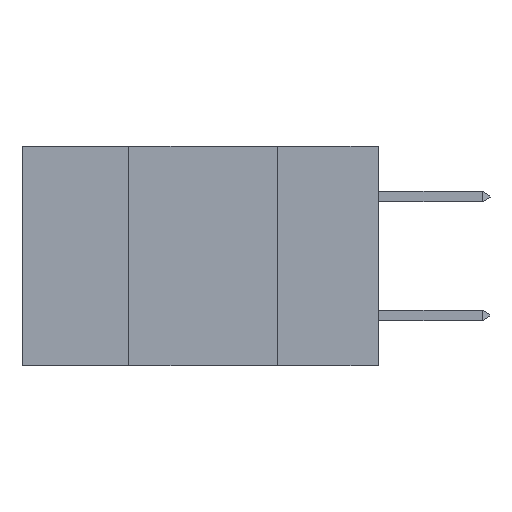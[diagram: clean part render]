
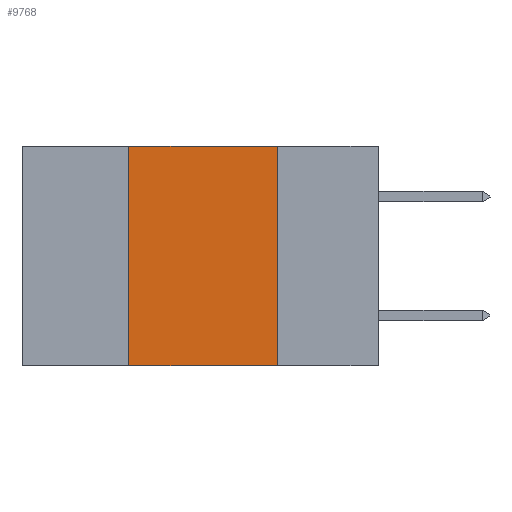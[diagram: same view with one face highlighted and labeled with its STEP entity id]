
A CAD part, left-side view. The second image highlights one B-rep face of the part: STEP entity #9768.
In plain terms, the highlighted planar face has unit normal (-1, 0, 0).
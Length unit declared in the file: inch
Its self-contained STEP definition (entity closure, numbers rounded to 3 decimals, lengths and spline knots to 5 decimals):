
#491 = VECTOR ( 'NONE', #6553, 39.37008 ) ;
#975 = DIRECTION ( 'NONE',  ( 1., 0., 0. ) ) ;
#2007 = LINE ( 'NONE', #8056, #9839 ) ;
#2958 = VERTEX_POINT ( 'NONE', #11075 ) ;
#3910 = CARTESIAN_POINT ( 'NONE',  ( 0., 0.17, 0. ) ) ;
#4146 = ORIENTED_EDGE ( 'NONE', *, *, #11691, .F. ) ;
#4901 = ORIENTED_EDGE ( 'NONE', *, *, #8458, .F. ) ;
#5192 = ORIENTED_EDGE ( 'NONE', *, *, #10136, .F. ) ;
#5673 = CARTESIAN_POINT ( 'NONE',  ( 0., 0.6, 0. ) ) ;
#5718 = ORIENTED_EDGE ( 'NONE', *, *, #8097, .T. ) ;
#6553 = DIRECTION ( 'NONE',  ( 0., 0., 1. ) ) ;
#8054 = LINE ( 'NONE', #3910, #19533 ) ;
#8056 = CARTESIAN_POINT ( 'NONE',  ( 0., 0.6, -0.37 ) ) ;
#8097 = EDGE_CURVE ( 'NONE', #2958, #17034, #2007, .T. ) ;
#8458 = EDGE_CURVE ( 'NONE', #16285, #9281, #15274, .T. ) ;
#8808 = LINE ( 'NONE', #11135, #491 ) ;
#9281 = VERTEX_POINT ( 'NONE', #12071 ) ;
#9768 = ADVANCED_FACE ( 'NONE', ( #11476 ), #10326, .F. ) ;
#9839 = VECTOR ( 'NONE', #15682, 39.37008 ) ;
#10136 = EDGE_CURVE ( 'NONE', #2958, #16285, #8808, .T. ) ;
#10326 = PLANE ( 'NONE',  #15379 ) ;
#10690 = EDGE_LOOP ( 'NONE', ( #4146, #4901, #5192, #5718 ) ) ;
#11075 = CARTESIAN_POINT ( 'NONE',  ( 0., 0.42, -0.37 ) ) ;
#11135 = CARTESIAN_POINT ( 'NONE',  ( 0., 0.42, 0. ) ) ;
#11476 = FACE_OUTER_BOUND ( 'NONE', #10690, .T. ) ;
#11691 = EDGE_CURVE ( 'NONE', #9281, #17034, #8054, .T. ) ;
#11860 = DIRECTION ( 'NONE',  ( 0., 0., -1. ) ) ;
#11973 = CARTESIAN_POINT ( 'NONE',  ( 0., 0.6, 0. ) ) ;
#12071 = CARTESIAN_POINT ( 'NONE',  ( 0., 0.17, 0. ) ) ;
#14637 = DIRECTION ( 'NONE',  ( 0., 0., -1. ) ) ;
#15274 = LINE ( 'NONE', #11973, #18733 ) ;
#15379 = AXIS2_PLACEMENT_3D ( 'NONE', #5673, #975, #11860 ) ;
#15682 = DIRECTION ( 'NONE',  ( 0., -1., 0. ) ) ;
#15936 = CARTESIAN_POINT ( 'NONE',  ( 0., 0.17, -0.37 ) ) ;
#16285 = VERTEX_POINT ( 'NONE', #17237 ) ;
#16510 = DIRECTION ( 'NONE',  ( 0., -1., 0. ) ) ;
#17034 = VERTEX_POINT ( 'NONE', #15936 ) ;
#17237 = CARTESIAN_POINT ( 'NONE',  ( 0., 0.42, 0. ) ) ;
#18733 = VECTOR ( 'NONE', #16510, 39.37008 ) ;
#19533 = VECTOR ( 'NONE', #14637, 39.37008 ) ;
